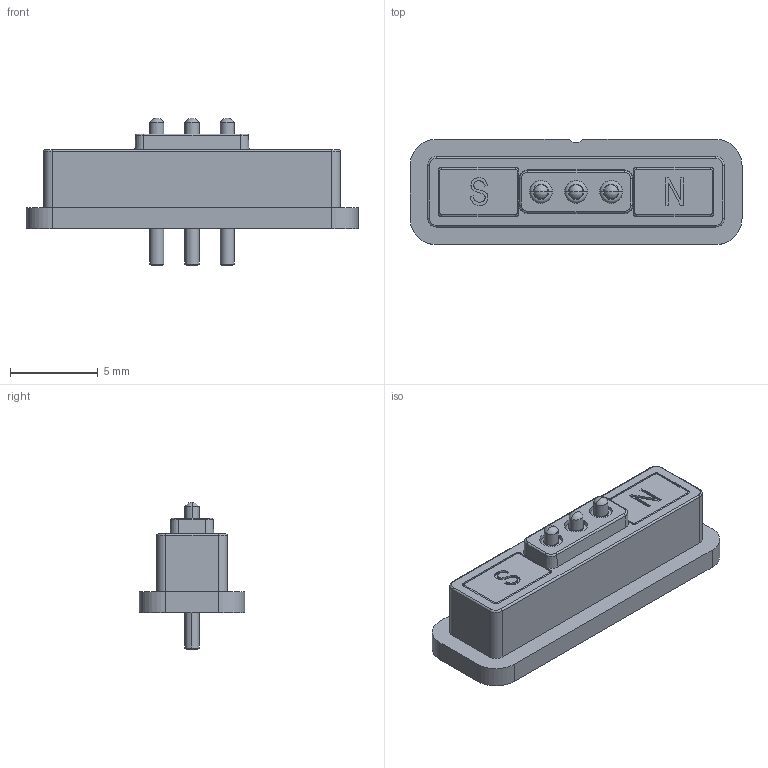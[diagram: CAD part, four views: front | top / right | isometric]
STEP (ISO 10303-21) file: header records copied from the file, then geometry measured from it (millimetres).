
FILE_DESCRIPTION (( 'STEP AP214' ), '1' );
FILE_NAME ('685F0321251110E.STEP', '2023-04-12T12:58:20', ( '' ), ( '' ), 'SwSTEP 2.0', 'SolidWorks 2020', '' );
FILE_SCHEMA (( 'AUTOMOTIVE_DESIGN' ));
Length unit declared in the file: millimetre
Products named in the file (1): 685F0321251110E
Bounding box: 18.9 x 6 x 8.4 mm (x, y, z)
Volume: 342.5 mm3; surface area: 621.1 mm2
Topology: 4 solids, 9 shells, 246 faces, 562 edges, 346 vertices
Faces by surface type: cylinder 93, plane 84, torus 30, cone 19, bspline 14, sphere 6
Entity records: 10280 total; most frequent: CARTESIAN_POINT 1985, DIRECTION 1245, ORIENTED_EDGE 1124, EDGE_CURVE 562, AXIS2_PLACEMENT_3D 478, VERTEX_POINT 346, VECTOR 289, LINE 289
